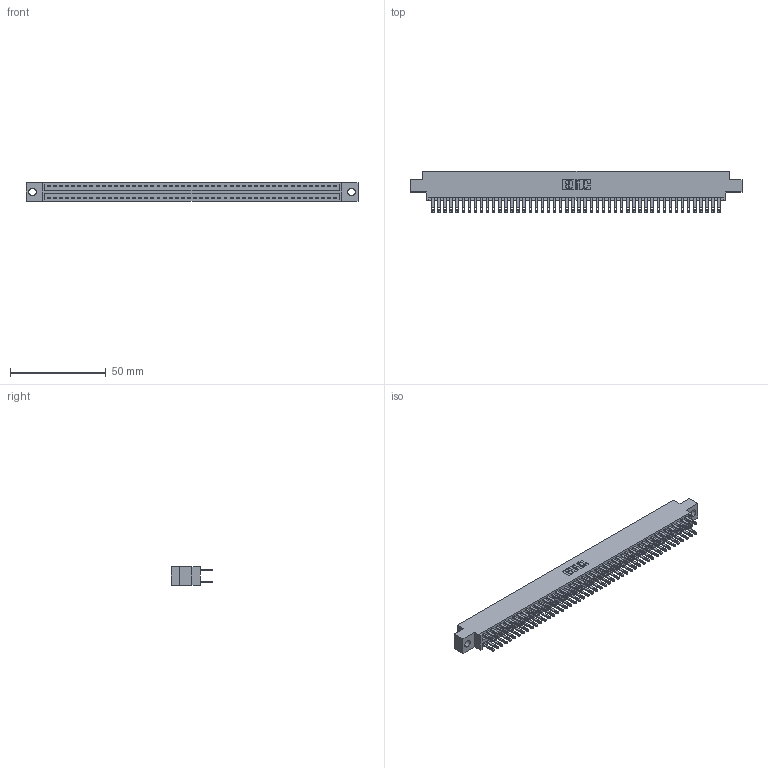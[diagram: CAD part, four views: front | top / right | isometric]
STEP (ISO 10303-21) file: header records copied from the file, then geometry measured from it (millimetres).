
FILE_DESCRIPTION (( 'STEP AP203' ), '1' );
FILE_NAME ('346-096-500-804.STEP', '2022-05-26T15:40:12', ( '' ), ( '' ), 'SwSTEP 2.0', 'SolidWorks 2020', '' );
FILE_SCHEMA (( 'CONFIG_CONTROL_DESIGN' ));
Length unit declared in the file: inch
Products named in the file (3): 346 Part_0.170 Offset - 0.156 Dia-TH; 345-292-001_345-293-100; 346-096-500-804
Assembly tree (97 placements, depth 2):
  346-096-500-804
    346 Part_0.170 Offset - 0.156 Dia-TH
    345-292-001_345-293-100  x96
Bounding box: 172.97 x 21.84 x 9.4 mm (x, y, z)
Volume: 16946.5 mm3; surface area: 24420.7 mm2
Topology: 97 solids, 97 shells, 4748 faces, 14489 edges, 9658 vertices
Faces by surface type: plane 2878, cylinder 1870
Entity records: 30999 total; most frequent: CARTESIAN_POINT 5106, ORIENTED_EDGE 5038, DIRECTION 4551, EDGE_CURVE 2519, VECTOR 2191, LINE 2191, VERTEX_POINT 1678, AXIS2_PLACEMENT_3D 1180
